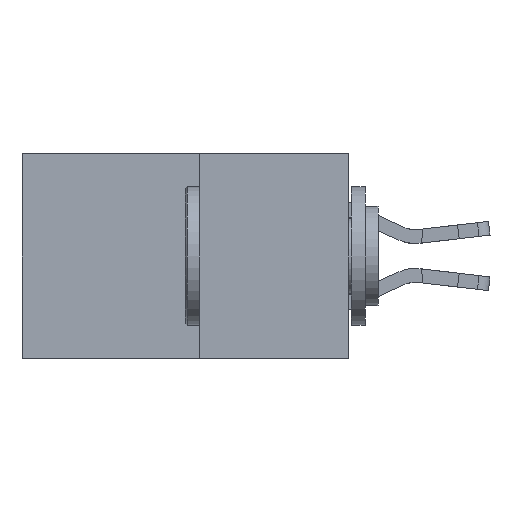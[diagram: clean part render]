
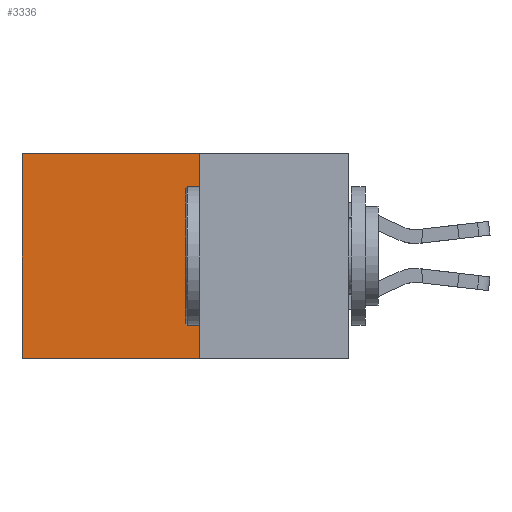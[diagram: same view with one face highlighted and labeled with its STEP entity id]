
A CAD part, left-side view. The second image highlights one B-rep face of the part: STEP entity #3336.
In plain terms, the highlighted planar face has unit normal (-1, 0, 0).
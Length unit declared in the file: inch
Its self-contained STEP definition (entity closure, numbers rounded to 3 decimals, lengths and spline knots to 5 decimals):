
#458 = VECTOR ( 'NONE', #2698, 39.37008 ) ;
#528 = EDGE_CURVE ( 'NONE', #21186, #30561, #24324, .T. ) ;
#781 = CARTESIAN_POINT ( 'NONE',  ( 0.277, 0.27, 0. ) ) ;
#2698 = DIRECTION ( 'NONE',  ( 0., 0., -1. ) ) ;
#2840 = CARTESIAN_POINT ( 'NONE',  ( 0.277, 0.27, -0.37 ) ) ;
#3221 = CARTESIAN_POINT ( 'NONE',  ( 0.277, 0.59, -0.37 ) ) ;
#3323 = DIRECTION ( 'NONE',  ( 0., 0., -1. ) ) ;
#3336 = ADVANCED_FACE ( 'NONE', ( #14600 ), #8760, .F. ) ;
#4157 = VECTOR ( 'NONE', #26815, 39.37008 ) ;
#6210 = ORIENTED_EDGE ( 'NONE', *, *, #14540, .F. ) ;
#6918 = LINE ( 'NONE', #3221, #26238 ) ;
#6998 = DIRECTION ( 'NONE',  ( 0., 0., -1. ) ) ;
#7078 = DIRECTION ( 'NONE',  ( 1., 0., 0. ) ) ;
#7386 = CARTESIAN_POINT ( 'NONE',  ( 0.277, 0.27, -0.37 ) ) ;
#8238 = EDGE_LOOP ( 'NONE', ( #25091, #31193, #6210, #25711 ) ) ;
#8614 = LINE ( 'NONE', #11208, #21325 ) ;
#8663 = CARTESIAN_POINT ( 'NONE',  ( 0.277, 0.59, 0. ) ) ;
#8760 = PLANE ( 'NONE',  #23920 ) ;
#9976 = EDGE_CURVE ( 'NONE', #20864, #22272, #8614, .T. ) ;
#11208 = CARTESIAN_POINT ( 'NONE',  ( 0.277, 0.27, -0.37 ) ) ;
#11560 = CARTESIAN_POINT ( 'NONE',  ( 0.277, 0.27, 0. ) ) ;
#13068 = CARTESIAN_POINT ( 'NONE',  ( 0.277, 0.59, -0.37 ) ) ;
#14540 = EDGE_CURVE ( 'NONE', #21186, #20864, #15530, .T. ) ;
#14600 = FACE_OUTER_BOUND ( 'NONE', #8238, .T. ) ;
#15471 = CARTESIAN_POINT ( 'NONE',  ( 0.277, 0.27, -0.37 ) ) ;
#15530 = LINE ( 'NONE', #15471, #458 ) ;
#18967 = EDGE_CURVE ( 'NONE', #30561, #22272, #6918, .T. ) ;
#20864 = VERTEX_POINT ( 'NONE', #2840 ) ;
#21186 = VERTEX_POINT ( 'NONE', #11560 ) ;
#21325 = VECTOR ( 'NONE', #31291, 39.37008 ) ;
#22272 = VERTEX_POINT ( 'NONE', #13068 ) ;
#23920 = AXIS2_PLACEMENT_3D ( 'NONE', #7386, #7078, #6998 ) ;
#24324 = LINE ( 'NONE', #781, #4157 ) ;
#25091 = ORIENTED_EDGE ( 'NONE', *, *, #18967, .T. ) ;
#25711 = ORIENTED_EDGE ( 'NONE', *, *, #528, .T. ) ;
#26238 = VECTOR ( 'NONE', #3323, 39.37008 ) ;
#26815 = DIRECTION ( 'NONE',  ( 0., 1., 0. ) ) ;
#30561 = VERTEX_POINT ( 'NONE', #8663 ) ;
#31193 = ORIENTED_EDGE ( 'NONE', *, *, #9976, .F. ) ;
#31291 = DIRECTION ( 'NONE',  ( 0., 1., 0. ) ) ;
